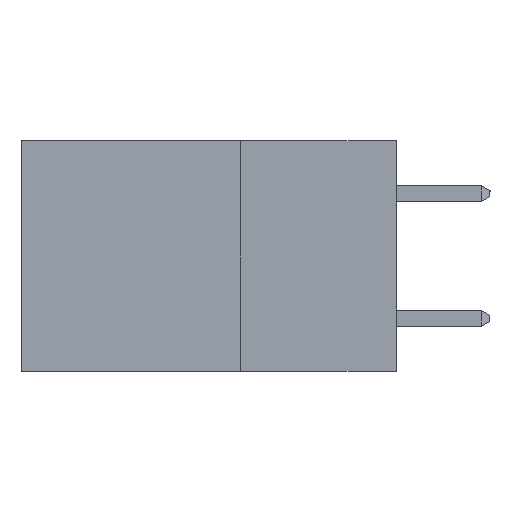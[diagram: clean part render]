
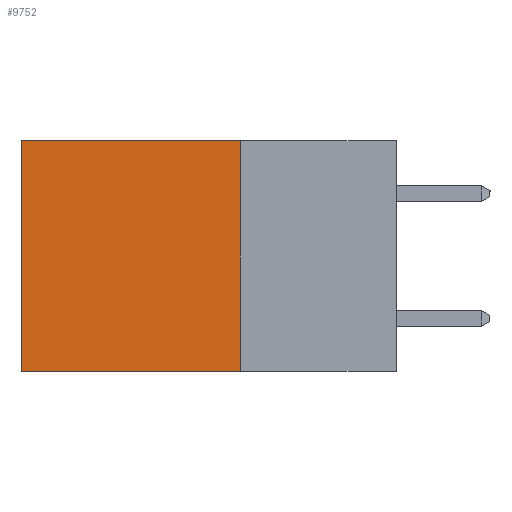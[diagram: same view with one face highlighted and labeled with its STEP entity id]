
A CAD part, left-side view. The second image highlights one B-rep face of the part: STEP entity #9752.
In plain terms, the highlighted planar face has unit normal (-1, 0, 0).
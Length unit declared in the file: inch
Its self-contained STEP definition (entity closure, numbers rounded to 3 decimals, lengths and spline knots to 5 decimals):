
#712 = VERTEX_POINT ( 'NONE', #13721 ) ;
#898 = VECTOR ( 'NONE', #13175, 39.37008 ) ;
#1274 = VECTOR ( 'NONE', #7696, 39.37008 ) ;
#1947 = CARTESIAN_POINT ( 'NONE',  ( 0.2615, 0.6, -0.37 ) ) ;
#2261 = VERTEX_POINT ( 'NONE', #12035 ) ;
#2273 = CARTESIAN_POINT ( 'NONE',  ( 0.2615, 0.25, 0. ) ) ;
#3080 = VERTEX_POINT ( 'NONE', #13167 ) ;
#3751 = EDGE_CURVE ( 'NONE', #2261, #8679, #14514, .T. ) ;
#4653 = CARTESIAN_POINT ( 'NONE',  ( 0.2615, 0.25, -0.37 ) ) ;
#4767 = ORIENTED_EDGE ( 'NONE', *, *, #7972, .F. ) ;
#5132 = EDGE_LOOP ( 'NONE', ( #11409, #6631, #4767, #6072 ) ) ;
#5220 = CARTESIAN_POINT ( 'NONE',  ( 0.2615, 0.6, -0.37 ) ) ;
#6024 = AXIS2_PLACEMENT_3D ( 'NONE', #8828, #13613, #12280 ) ;
#6072 = ORIENTED_EDGE ( 'NONE', *, *, #13475, .T. ) ;
#6631 = ORIENTED_EDGE ( 'NONE', *, *, #14721, .F. ) ;
#6898 = LINE ( 'NONE', #2273, #10875 ) ;
#7696 = DIRECTION ( 'NONE',  ( 0., 0., -1. ) ) ;
#7972 = EDGE_CURVE ( 'NONE', #3080, #712, #11454, .T. ) ;
#8325 = DIRECTION ( 'NONE',  ( 0., 0., -1. ) ) ;
#8625 = CARTESIAN_POINT ( 'NONE',  ( 0.2615, 0.25, -0.37 ) ) ;
#8679 = VERTEX_POINT ( 'NONE', #5220 ) ;
#8828 = CARTESIAN_POINT ( 'NONE',  ( 0.2615, 0.25, -0.37 ) ) ;
#9115 = VECTOR ( 'NONE', #8325, 39.37008 ) ;
#9741 = LINE ( 'NONE', #8625, #898 ) ;
#9752 = ADVANCED_FACE ( 'NONE', ( #9960 ), #10180, .F. ) ;
#9960 = FACE_OUTER_BOUND ( 'NONE', #5132, .T. ) ;
#10180 = PLANE ( 'NONE',  #6024 ) ;
#10875 = VECTOR ( 'NONE', #12573, 39.37008 ) ;
#11409 = ORIENTED_EDGE ( 'NONE', *, *, #3751, .T. ) ;
#11454 = LINE ( 'NONE', #4653, #9115 ) ;
#12035 = CARTESIAN_POINT ( 'NONE',  ( 0.2615, 0.6, 0. ) ) ;
#12280 = DIRECTION ( 'NONE',  ( 0., 0., -1. ) ) ;
#12573 = DIRECTION ( 'NONE',  ( 0., 1., 0. ) ) ;
#13167 = CARTESIAN_POINT ( 'NONE',  ( 0.2615, 0.25, 0. ) ) ;
#13175 = DIRECTION ( 'NONE',  ( 0., 1., 0. ) ) ;
#13475 = EDGE_CURVE ( 'NONE', #3080, #2261, #6898, .T. ) ;
#13613 = DIRECTION ( 'NONE',  ( 1., 0., 0. ) ) ;
#13721 = CARTESIAN_POINT ( 'NONE',  ( 0.2615, 0.25, -0.37 ) ) ;
#14514 = LINE ( 'NONE', #1947, #1274 ) ;
#14721 = EDGE_CURVE ( 'NONE', #712, #8679, #9741, .T. ) ;
